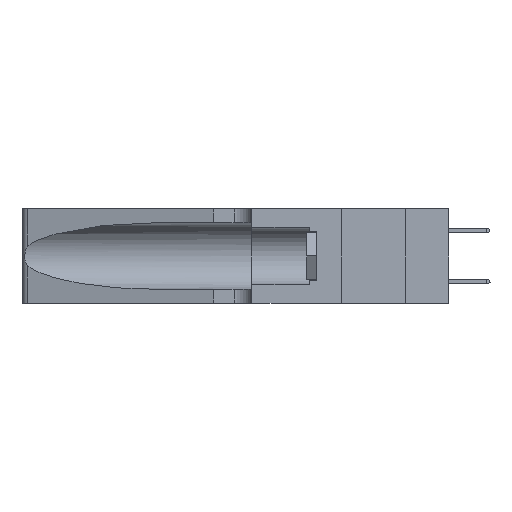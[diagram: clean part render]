
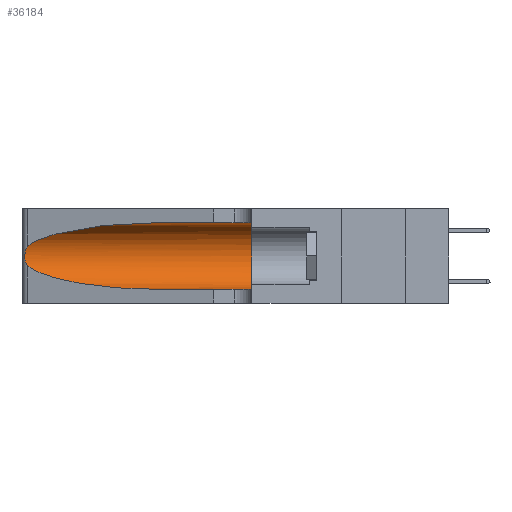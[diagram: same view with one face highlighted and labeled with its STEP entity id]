
A CAD part, left-side view. The second image highlights one B-rep face of the part: STEP entity #36184.
In plain terms, the highlighted cylindrical face has radius 3.308 mm (diameter 6.617 mm), a partial arc.
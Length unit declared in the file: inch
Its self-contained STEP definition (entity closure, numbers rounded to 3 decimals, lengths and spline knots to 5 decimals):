
#37 = CARTESIAN_POINT ( 'NONE',  ( 0.25487, 1.22718, 0.22369 ) ) ;
#444 = VERTEX_POINT ( 'NONE', #36911 ) ;
#1269 = CARTESIAN_POINT ( 'NONE',  ( 0.1305, 1.61858, 0.05475 ) ) ;
#2822 = CARTESIAN_POINT ( 'NONE',  ( 0.25787, 1.23484, 0.2124 ) ) ;
#4646 = DIRECTION ( 'NONE',  ( 0., -1., 0. ) ) ;
#4738 = CARTESIAN_POINT ( 'NONE',  ( 0.18966, 0.96281, 0.05475 ) ) ;
#5536 = EDGE_CURVE ( 'NONE', #5733, #444, #22878, .T. ) ;
#5733 = VERTEX_POINT ( 'NONE', #7687 ) ;
#5975 = EDGE_CURVE ( 'NONE', #5733, #25953, #16847, .T. ) ;
#6202 = CARTESIAN_POINT ( 'NONE',  ( 0.26018, 1.23835, 0.19895 ) ) ;
#6933 = DIRECTION ( 'NONE',  ( 0., 1., 0. ) ) ;
#7687 = CARTESIAN_POINT ( 'NONE',  ( 0.1305, 0.72297, 0.31525 ) ) ;
#7958 = CARTESIAN_POINT ( 'NONE',  ( 0.25487, 1.22718, 0.14631 ) ) ;
#8702 = VERTEX_POINT ( 'NONE', #35470 ) ;
#9006 = CARTESIAN_POINT ( 'NONE',  ( 0.1305, 1.61858, 0.31525 ) ) ;
#9615 = CARTESIAN_POINT ( 'NONE',  ( 0.26075, 1.23896, 0.178 ) ) ;
#11652 = EDGE_CURVE ( 'NONE', #30262, #8702, #40669, .T. ) ;
#11751 = EDGE_LOOP ( 'NONE', ( #25603, #18683, #27156, #29038, #14803, #34161 ) ) ;
#12380 = DIRECTION ( 'NONE',  ( 0., -1., 0. ) ) ;
#12980 = CARTESIAN_POINT ( 'NONE',  ( 0.25856, 1.23593, 0.16098 ) ) ;
#13632 = VERTEX_POINT ( 'NONE', #7958 ) ;
#14803 = ORIENTED_EDGE ( 'NONE', *, *, #19619, .F. ) ;
#16184 = CARTESIAN_POINT ( 'NONE',  ( 0.25555, 1.22994, 0.2215 ) ) ;
#16314 = CARTESIAN_POINT ( 'NONE',  ( 0.25639, 1.23186, 0.15144 ) ) ;
#16779 = CARTESIAN_POINT ( 'NONE',  ( 0.18966, 0.96281, 0.31525 ) ) ;
#16847 = LINE ( 'NONE', #9006, #41225 ) ;
#18683 = ORIENTED_EDGE ( 'NONE', *, *, #33282, .T. ) ;
#18742 = DIRECTION ( 'NONE',  ( 0., -1., 0. ) ) ;
#19557 = CARTESIAN_POINT ( 'NONE',  ( 0.25487, 1.22718, 0.22369 ) ) ;
#19619 = EDGE_CURVE ( 'NONE', #25953, #8702, #31982, .T. ) ;
#19693 = B_SPLINE_CURVE_WITH_KNOTS ( 'NONE', 3,
 ( #19557, #16184, #22882, #2822, #26202, #6202, #29536, #9615, #32881, #12980, #36223, #16314, #39531, #19696 ),
 .UNSPECIFIED., .F., .F.,
 ( 4, 2, 2, 2, 2, 2, 4 ),
 ( 0., 0.00027, 0.00053, 0.00107, 0.0016, 0.00187, 0.00214 ),
 .UNSPECIFIED. ) ;
#19696 = CARTESIAN_POINT ( 'NONE',  ( 0.25487, 1.22718, 0.14631 ) ) ;
#20144 = CARTESIAN_POINT ( 'NONE',  ( 0.2373, 1.15595, 0.28018 ) ) ;
#20327 = CYLINDRICAL_SURFACE ( 'NONE', #25330, 0.13025 ) ;
#21454 = CARTESIAN_POINT ( 'NONE',  ( 0.25487, 1.22718, 0.14631 ) ) ;
#22029 = VECTOR ( 'NONE', #4646, 39.37008 ) ;
#22878 =( BOUNDED_CURVE ( )  B_SPLINE_CURVE ( 3, ( #39967, #16779, #20144, #37 ),
 .UNSPECIFIED., .F., .F. ) 
 B_SPLINE_CURVE_WITH_KNOTS ( ( 4, 4 ),
 ( 1.5708, 2.84003 ),
 .UNSPECIFIED. ) 
 CURVE ( )  GEOMETRIC_REPRESENTATION_ITEM ( )  RATIONAL_B_SPLINE_CURVE ( ( 1., 0.87, 0.87, 1. ) ) 
 REPRESENTATION_ITEM ( '' )  );
#22882 = CARTESIAN_POINT ( 'NONE',  ( 0.25639, 1.23184, 0.21858 ) ) ;
#24772 = CARTESIAN_POINT ( 'NONE',  ( 0.2373, 1.15595, 0.08982 ) ) ;
#25330 = AXIS2_PLACEMENT_3D ( 'NONE', #35276, #18742, #41911 ) ;
#25603 = ORIENTED_EDGE ( 'NONE', *, *, #5536, .T. ) ;
#25953 = VERTEX_POINT ( 'NONE', #26079 ) ;
#26079 = CARTESIAN_POINT ( 'NONE',  ( 0.1305, 0.35, 0.31525 ) ) ;
#26202 = CARTESIAN_POINT ( 'NONE',  ( 0.25854, 1.2359, 0.20912 ) ) ;
#26918 = CARTESIAN_POINT ( 'NONE',  ( 0.1305, 0.35, 0.185 ) ) ;
#27156 = ORIENTED_EDGE ( 'NONE', *, *, #33018, .T. ) ;
#27386 =( BOUNDED_CURVE ( )  B_SPLINE_CURVE ( 3, ( #21454, #24772, #4738, #28135 ),
 .UNSPECIFIED., .F., .F. ) 
 B_SPLINE_CURVE_WITH_KNOTS ( ( 4, 4 ),
 ( 3.44316, 4.71239 ),
 .UNSPECIFIED. ) 
 CURVE ( )  GEOMETRIC_REPRESENTATION_ITEM ( )  RATIONAL_B_SPLINE_CURVE ( ( 1., 0.87, 0.87, 1. ) ) 
 REPRESENTATION_ITEM ( '' )  );
#28135 = CARTESIAN_POINT ( 'NONE',  ( 0.1305, 0.72297, 0.05475 ) ) ;
#29038 = ORIENTED_EDGE ( 'NONE', *, *, #11652, .T. ) ;
#29536 = CARTESIAN_POINT ( 'NONE',  ( 0.26075, 1.23896, 0.19203 ) ) ;
#30182 = FACE_OUTER_BOUND ( 'NONE', #11751, .T. ) ;
#30262 = VERTEX_POINT ( 'NONE', #34038 ) ;
#30273 = DIRECTION ( 'NONE',  ( 0., 0., 1. ) ) ;
#31982 = CIRCLE ( 'NONE', #42144, 0.13025 ) ;
#32881 = CARTESIAN_POINT ( 'NONE',  ( 0.26017, 1.23833, 0.17102 ) ) ;
#33018 = EDGE_CURVE ( 'NONE', #13632, #30262, #27386, .T. ) ;
#33282 = EDGE_CURVE ( 'NONE', #444, #13632, #19693, .T. ) ;
#34038 = CARTESIAN_POINT ( 'NONE',  ( 0.1305, 0.72297, 0.05475 ) ) ;
#34161 = ORIENTED_EDGE ( 'NONE', *, *, #5975, .F. ) ;
#35276 = CARTESIAN_POINT ( 'NONE',  ( 0.1305, 1.61858, 0.185 ) ) ;
#35470 = CARTESIAN_POINT ( 'NONE',  ( 0.1305, 0.35, 0.05475 ) ) ;
#36184 = ADVANCED_FACE ( 'NONE', ( #30182 ), #20327, .F. ) ;
#36223 = CARTESIAN_POINT ( 'NONE',  ( 0.25789, 1.23486, 0.15765 ) ) ;
#36911 = CARTESIAN_POINT ( 'NONE',  ( 0.25487, 1.22718, 0.22369 ) ) ;
#39531 = CARTESIAN_POINT ( 'NONE',  ( 0.25555, 1.22993, 0.14849 ) ) ;
#39967 = CARTESIAN_POINT ( 'NONE',  ( 0.1305, 0.72297, 0.31525 ) ) ;
#40669 = LINE ( 'NONE', #1269, #22029 ) ;
#41225 = VECTOR ( 'NONE', #12380, 39.37008 ) ;
#41911 = DIRECTION ( 'NONE',  ( 0., 0., -1. ) ) ;
#42144 = AXIS2_PLACEMENT_3D ( 'NONE', #26918, #6933, #30273 ) ;
